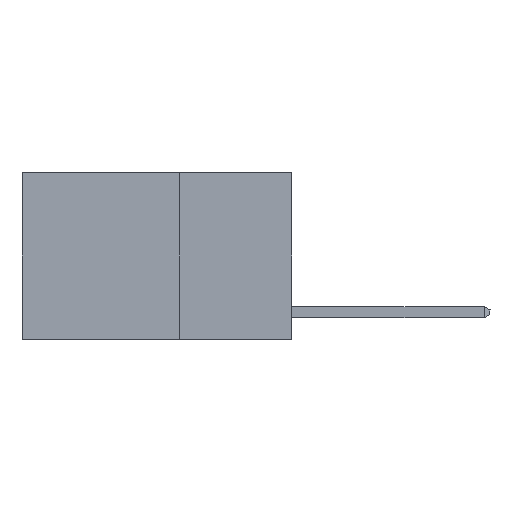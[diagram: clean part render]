
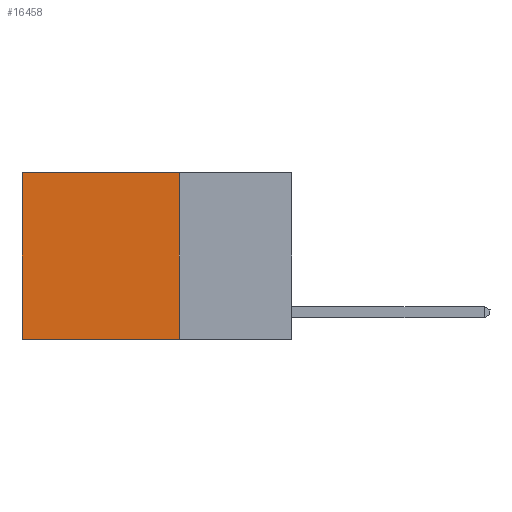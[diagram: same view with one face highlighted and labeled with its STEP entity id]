
A CAD part, left-side view. The second image highlights one B-rep face of the part: STEP entity #16458.
In plain terms, the highlighted planar face has unit normal (-1, 0, 0).
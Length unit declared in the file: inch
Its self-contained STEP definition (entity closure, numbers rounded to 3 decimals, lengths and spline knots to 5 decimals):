
#370 = DIRECTION ( 'NONE',  ( 0., 0., -1. ) ) ;
#467 = DIRECTION ( 'NONE',  ( 0., 0., -1. ) ) ;
#1572 = ORIENTED_EDGE ( 'NONE', *, *, #16844, .T. ) ;
#2657 = CARTESIAN_POINT ( 'NONE',  ( 0.2625, 0.25, 0. ) ) ;
#3414 = CARTESIAN_POINT ( 'NONE',  ( 0.2625, 0.25, -0.37 ) ) ;
#3862 = CARTESIAN_POINT ( 'NONE',  ( 0.2625, 0.6, 0. ) ) ;
#3929 = VECTOR ( 'NONE', #11393, 39.37008 ) ;
#4928 = VECTOR ( 'NONE', #15386, 39.37008 ) ;
#5158 = VERTEX_POINT ( 'NONE', #3862 ) ;
#5351 = AXIS2_PLACEMENT_3D ( 'NONE', #12024, #22060, #370 ) ;
#6027 = CARTESIAN_POINT ( 'NONE',  ( 0.2625, 0.6, -0.37 ) ) ;
#7252 = EDGE_CURVE ( 'NONE', #15423, #19993, #20054, .T. ) ;
#10380 = VERTEX_POINT ( 'NONE', #6027 ) ;
#10963 = EDGE_CURVE ( 'NONE', #15423, #5158, #18336, .T. ) ;
#11393 = DIRECTION ( 'NONE',  ( 0., 0., -1. ) ) ;
#11530 = ORIENTED_EDGE ( 'NONE', *, *, #7252, .F. ) ;
#12024 = CARTESIAN_POINT ( 'NONE',  ( 0.2625, 0.25, 0. ) ) ;
#14264 = ORIENTED_EDGE ( 'NONE', *, *, #15667, .F. ) ;
#14872 = VECTOR ( 'NONE', #467, 39.37008 ) ;
#15386 = DIRECTION ( 'NONE',  ( 0., 1., 0. ) ) ;
#15423 = VERTEX_POINT ( 'NONE', #2657 ) ;
#15477 = FACE_OUTER_BOUND ( 'NONE', #22619, .T. ) ;
#15667 = EDGE_CURVE ( 'NONE', #19993, #10380, #23211, .T. ) ;
#16458 = ADVANCED_FACE ( 'NONE', ( #15477 ), #20039, .F. ) ;
#16844 = EDGE_CURVE ( 'NONE', #5158, #10380, #23754, .T. ) ;
#17519 = CARTESIAN_POINT ( 'NONE',  ( 0.2625, 0.25, -0.37 ) ) ;
#18081 = CARTESIAN_POINT ( 'NONE',  ( 0.2625, 0.25, 0. ) ) ;
#18336 = LINE ( 'NONE', #22666, #20170 ) ;
#18923 = ORIENTED_EDGE ( 'NONE', *, *, #10963, .T. ) ;
#19993 = VERTEX_POINT ( 'NONE', #17519 ) ;
#20039 = PLANE ( 'NONE',  #5351 ) ;
#20054 = LINE ( 'NONE', #18081, #14872 ) ;
#20170 = VECTOR ( 'NONE', #22754, 39.37008 ) ;
#21166 = CARTESIAN_POINT ( 'NONE',  ( 0.2625, 0.6, 0. ) ) ;
#22060 = DIRECTION ( 'NONE',  ( 1., 0., 0. ) ) ;
#22619 = EDGE_LOOP ( 'NONE', ( #1572, #14264, #11530, #18923 ) ) ;
#22666 = CARTESIAN_POINT ( 'NONE',  ( 0.2625, 0.25, 0. ) ) ;
#22754 = DIRECTION ( 'NONE',  ( 0., 1., 0. ) ) ;
#23211 = LINE ( 'NONE', #3414, #4928 ) ;
#23754 = LINE ( 'NONE', #21166, #3929 ) ;
